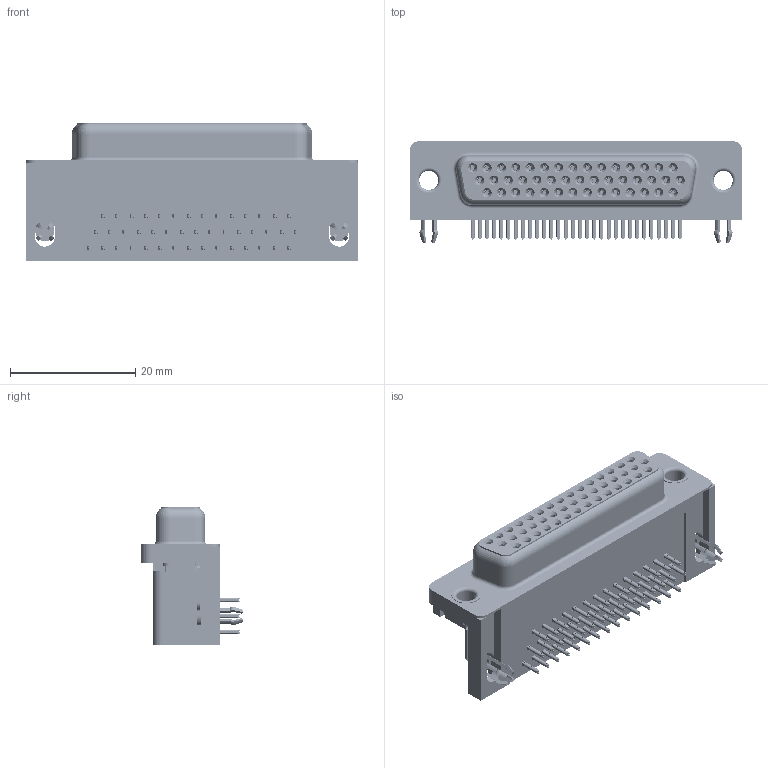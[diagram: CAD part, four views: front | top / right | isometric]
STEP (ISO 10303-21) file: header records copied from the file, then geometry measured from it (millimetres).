
FILE_DESCRIPTION (( 'STEP AP203' ), '1' );
FILE_NAME ('634-044-663-541.STEP', '2018-11-10T01:22:17', ( '' ), ( '' ), 'SwSTEP 2.0', 'SolidWorks 2016', '' );
FILE_SCHEMA (( 'CONFIG_CONTROL_DESIGN' ));
Length unit declared in the file: millimetre
Products named in the file (8): Contact Middle; Contact Top; 4 Prong Board Lock; Thru Hole Rivet; 634-044-663-541; 634 Housing_44 Socket; 634 Shell_44 Socket; Contact Bottom
Assembly tree (50 placements, depth 2):
  634-044-663-541
    634 Housing_44 Socket
    634 Shell_44 Socket
    Contact Bottom  x14
    Contact Middle  x15
    Contact Top  x15
    4 Prong Board Lock  x2
    Thru Hole Rivet  x2
Bounding box: 53.04 x 16.25 x 22.1 mm (x, y, z)
Volume: 9354.6 mm3; surface area: 13334.7 mm2
Topology: 50 solids, 50 shells, 6617 faces, 17430 edges, 10950 vertices
Faces by surface type: plane 2971, bspline 1528, cylinder 1484, cone 568, torus 66
Entity records: 44525 total; most frequent: CARTESIAN_POINT 12041, ORIENTED_EDGE 6430, DIRECTION 6004, EDGE_CURVE 3215, VECTOR 2158, LINE 2158, VERTEX_POINT 2058, AXIS2_PLACEMENT_3D 1923
